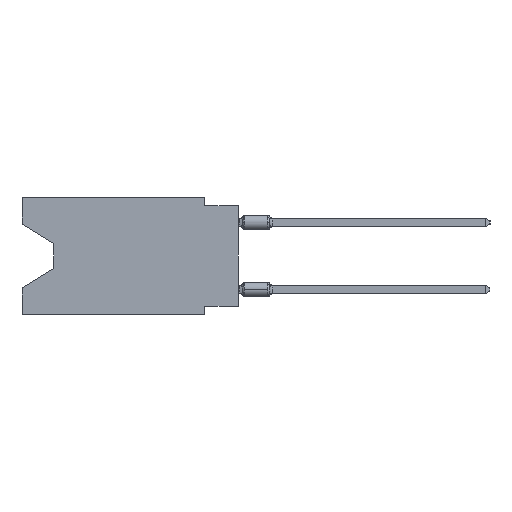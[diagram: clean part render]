
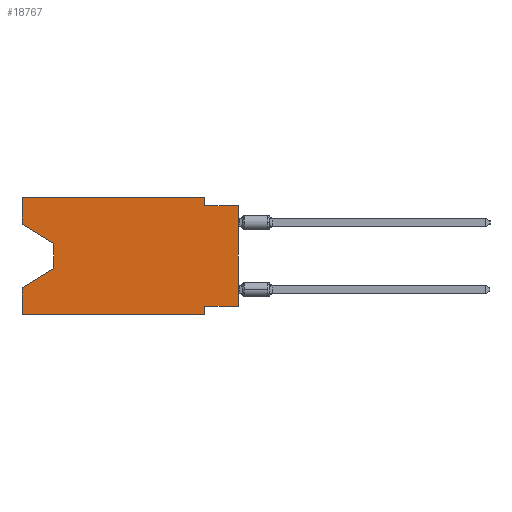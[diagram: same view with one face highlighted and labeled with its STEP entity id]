
A CAD part, left-side view. The second image highlights one B-rep face of the part: STEP entity #18767.
In plain terms, the highlighted planar face has unit normal (-1, 0, 0).
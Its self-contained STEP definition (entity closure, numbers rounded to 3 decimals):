
#604 = EDGE_CURVE ( 'NONE', #22103, #11759, #44241, .T. ) ;
#697 = CARTESIAN_POINT ( 'NONE',  ( 0., 16.383, 0. ) ) ;
#805 = VECTOR ( 'NONE', #17674, 1000. ) ;
#1069 = VERTEX_POINT ( 'NONE', #51786 ) ;
#1704 = LINE ( 'NONE', #50729, #46278 ) ;
#1879 = LINE ( 'NONE', #10157, #51346 ) ;
#2659 = VECTOR ( 'NONE', #32347, 1000. ) ;
#2737 = DIRECTION ( 'NONE',  ( 0., -1., 0. ) ) ;
#2808 = DIRECTION ( 'NONE',  ( 0., 0., -1. ) ) ;
#3143 = CARTESIAN_POINT ( 'NONE',  ( 0., 16.383, -2.038 ) ) ;
#4224 = LINE ( 'NONE', #48546, #44987 ) ;
#4302 = CARTESIAN_POINT ( 'NONE',  ( 0., 13.97, -3.505 ) ) ;
#5215 = EDGE_LOOP ( 'NONE', ( #37118, #7252, #34432, #26094, #56132, #56543, #35363, #5458, #27886, #56221, #44074, #23146 ) ) ;
#5315 = VECTOR ( 'NONE', #32286, 1000. ) ;
#5458 = ORIENTED_EDGE ( 'NONE', *, *, #16909, .T. ) ;
#5750 = VERTEX_POINT ( 'NONE', #16632 ) ;
#5830 = VERTEX_POINT ( 'NONE', #21054 ) ;
#7067 = CARTESIAN_POINT ( 'NONE',  ( 0., 16.383, -6.852 ) ) ;
#7252 = ORIENTED_EDGE ( 'NONE', *, *, #10634, .T. ) ;
#7682 = VERTEX_POINT ( 'NONE', #7067 ) ;
#8292 = EDGE_CURVE ( 'NONE', #10908, #11012, #18470, .T. ) ;
#8388 = EDGE_CURVE ( 'NONE', #10908, #55993, #56240, .T. ) ;
#9097 = LINE ( 'NONE', #44824, #56614 ) ;
#9603 = CARTESIAN_POINT ( 'NONE',  ( 0., 16.383, -2.038 ) ) ;
#10157 = CARTESIAN_POINT ( 'NONE',  ( 0., 16.383, 0. ) ) ;
#10479 = DIRECTION ( 'NONE',  ( 0., 0., 1. ) ) ;
#10634 = EDGE_CURVE ( 'NONE', #11012, #57410, #9097, .T. ) ;
#10837 = EDGE_CURVE ( 'NONE', #5750, #5830, #1704, .T. ) ;
#10908 = VERTEX_POINT ( 'NONE', #3143 ) ;
#11012 = VERTEX_POINT ( 'NONE', #4302 ) ;
#11432 = VECTOR ( 'NONE', #2808, 1000. ) ;
#11468 = CARTESIAN_POINT ( 'NONE',  ( 0., 2.54, 0. ) ) ;
#11759 = VERTEX_POINT ( 'NONE', #56744 ) ;
#11925 = EDGE_CURVE ( 'NONE', #57410, #7682, #54361, .T. ) ;
#12571 = EDGE_CURVE ( 'NONE', #44061, #1069, #21394, .T. ) ;
#14546 = AXIS2_PLACEMENT_3D ( 'NONE', #24768, #51653, #42203 ) ;
#16254 = VERTEX_POINT ( 'NONE', #41713 ) ;
#16375 = EDGE_CURVE ( 'NONE', #5750, #7682, #45556, .T. ) ;
#16632 = CARTESIAN_POINT ( 'NONE',  ( 0., 16.383, -8.89 ) ) ;
#16671 = DIRECTION ( 'NONE',  ( 0., 1., 0. ) ) ;
#16900 = CARTESIAN_POINT ( 'NONE',  ( 0., 0., -0.635 ) ) ;
#16909 = EDGE_CURVE ( 'NONE', #44061, #16254, #4224, .T. ) ;
#17168 = CARTESIAN_POINT ( 'NONE',  ( 0., 13.97, -5.385 ) ) ;
#17529 = DIRECTION ( 'NONE',  ( 0., 0., 1. ) ) ;
#17674 = DIRECTION ( 'NONE',  ( 0., 0., -1. ) ) ;
#17754 = VECTOR ( 'NONE', #10479, 1000. ) ;
#18373 = CARTESIAN_POINT ( 'NONE',  ( 0., 13.97, -5.385 ) ) ;
#18470 = LINE ( 'NONE', #9603, #2659 ) ;
#18767 = ADVANCED_FACE ( 'NONE', ( #28614 ), #50773, .F. ) ;
#19709 = DIRECTION ( 'NONE',  ( 0., -1., 0. ) ) ;
#20907 = VECTOR ( 'NONE', #2737, 1000. ) ;
#21054 = CARTESIAN_POINT ( 'NONE',  ( 0., 2.54, -8.89 ) ) ;
#21394 = LINE ( 'NONE', #53276, #47215 ) ;
#22091 = CARTESIAN_POINT ( 'NONE',  ( 0., 2.54, 0. ) ) ;
#22103 = VERTEX_POINT ( 'NONE', #11468 ) ;
#23146 = ORIENTED_EDGE ( 'NONE', *, *, #8388, .F. ) ;
#24768 = CARTESIAN_POINT ( 'NONE',  ( 0., 16.383, 0. ) ) ;
#26094 = ORIENTED_EDGE ( 'NONE', *, *, #16375, .F. ) ;
#27886 = ORIENTED_EDGE ( 'NONE', *, *, #55986, .F. ) ;
#28614 = FACE_OUTER_BOUND ( 'NONE', #5215, .T. ) ;
#29611 = LINE ( 'NONE', #16900, #20907 ) ;
#32286 = DIRECTION ( 'NONE',  ( 0., 0., 1. ) ) ;
#32347 = DIRECTION ( 'NONE',  ( 0., -0.855, -0.519 ) ) ;
#33488 = DIRECTION ( 'NONE',  ( 0., -1., 0. ) ) ;
#34432 = ORIENTED_EDGE ( 'NONE', *, *, #11925, .T. ) ;
#35363 = ORIENTED_EDGE ( 'NONE', *, *, #12571, .F. ) ;
#35768 = DIRECTION ( 'NONE',  ( 0., 0.855, -0.519 ) ) ;
#37118 = ORIENTED_EDGE ( 'NONE', *, *, #8292, .T. ) ;
#41270 = DIRECTION ( 'NONE',  ( 0., 0., -1. ) ) ;
#41713 = CARTESIAN_POINT ( 'NONE',  ( 0., 0., -0.635 ) ) ;
#42203 = DIRECTION ( 'NONE',  ( 0., 0., -1. ) ) ;
#43483 = CARTESIAN_POINT ( 'NONE',  ( 0., 16.383, 0. ) ) ;
#44061 = VERTEX_POINT ( 'NONE', #47428 ) ;
#44074 = ORIENTED_EDGE ( 'NONE', *, *, #51024, .F. ) ;
#44138 = CARTESIAN_POINT ( 'NONE',  ( 0., 2.54, -8.89 ) ) ;
#44241 = LINE ( 'NONE', #22091, #805 ) ;
#44824 = CARTESIAN_POINT ( 'NONE',  ( 0., 13.97, -3.505 ) ) ;
#44987 = VECTOR ( 'NONE', #17529, 1000. ) ;
#45556 = LINE ( 'NONE', #697, #5315 ) ;
#46278 = VECTOR ( 'NONE', #19709, 1000. ) ;
#46801 = CARTESIAN_POINT ( 'NONE',  ( 0., 16.383, 0. ) ) ;
#47215 = VECTOR ( 'NONE', #16671, 1000. ) ;
#47428 = CARTESIAN_POINT ( 'NONE',  ( 0., 0., -8.255 ) ) ;
#48546 = CARTESIAN_POINT ( 'NONE',  ( 0., 0., 0. ) ) ;
#50729 = CARTESIAN_POINT ( 'NONE',  ( 0., 16.383, -8.89 ) ) ;
#50773 = PLANE ( 'NONE',  #14546 ) ;
#51024 = EDGE_CURVE ( 'NONE', #55993, #22103, #1879, .T. ) ;
#51346 = VECTOR ( 'NONE', #33488, 1000. ) ;
#51653 = DIRECTION ( 'NONE',  ( 1., 0., 0. ) ) ;
#51786 = CARTESIAN_POINT ( 'NONE',  ( 0., 2.54, -8.255 ) ) ;
#53276 = CARTESIAN_POINT ( 'NONE',  ( 0., 0., -8.255 ) ) ;
#54361 = LINE ( 'NONE', #17168, #57532 ) ;
#55529 = EDGE_CURVE ( 'NONE', #1069, #5830, #57712, .T. ) ;
#55986 = EDGE_CURVE ( 'NONE', #11759, #16254, #29611, .T. ) ;
#55993 = VERTEX_POINT ( 'NONE', #43483 ) ;
#56132 = ORIENTED_EDGE ( 'NONE', *, *, #10837, .T. ) ;
#56221 = ORIENTED_EDGE ( 'NONE', *, *, #604, .F. ) ;
#56240 = LINE ( 'NONE', #46801, #17754 ) ;
#56543 = ORIENTED_EDGE ( 'NONE', *, *, #55529, .F. ) ;
#56614 = VECTOR ( 'NONE', #41270, 1000. ) ;
#56744 = CARTESIAN_POINT ( 'NONE',  ( 0., 2.54, -0.635 ) ) ;
#57410 = VERTEX_POINT ( 'NONE', #18373 ) ;
#57532 = VECTOR ( 'NONE', #35768, 1000. ) ;
#57712 = LINE ( 'NONE', #44138, #11432 ) ;
